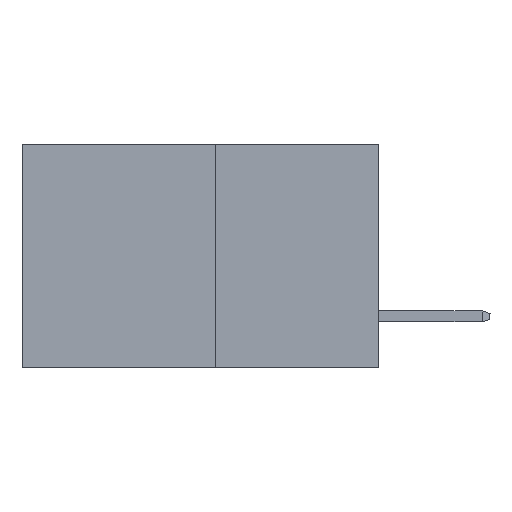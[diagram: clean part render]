
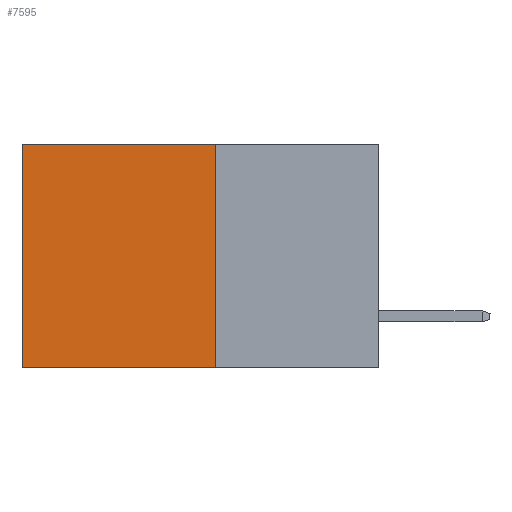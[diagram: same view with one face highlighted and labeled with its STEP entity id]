
A CAD part, left-side view. The second image highlights one B-rep face of the part: STEP entity #7595.
In plain terms, the highlighted planar face has unit normal (-1, 0, 0).
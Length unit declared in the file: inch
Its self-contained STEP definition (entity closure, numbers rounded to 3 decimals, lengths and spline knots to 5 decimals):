
#666 = CARTESIAN_POINT ( 'NONE',  ( 0.277, 0.59, -0.37 ) ) ;
#1176 = ORIENTED_EDGE ( 'NONE', *, *, #9642, .T. ) ;
#1651 = DIRECTION ( 'NONE',  ( 1., 0., 0. ) ) ;
#1742 = CARTESIAN_POINT ( 'NONE',  ( 0.277, 0.27, -0.37 ) ) ;
#2065 = LINE ( 'NONE', #10986, #4823 ) ;
#2217 = VECTOR ( 'NONE', #12589, 39.37008 ) ;
#2310 = EDGE_CURVE ( 'NONE', #8535, #12122, #2065, .T. ) ;
#2822 = CARTESIAN_POINT ( 'NONE',  ( 0.277, 0.59, 0. ) ) ;
#3288 = EDGE_CURVE ( 'NONE', #3587, #8535, #10731, .T. ) ;
#3301 = ORIENTED_EDGE ( 'NONE', *, *, #3288, .F. ) ;
#3587 = VERTEX_POINT ( 'NONE', #5481 ) ;
#4823 = VECTOR ( 'NONE', #12206, 39.37008 ) ;
#5037 = FACE_OUTER_BOUND ( 'NONE', #9085, .T. ) ;
#5169 = VECTOR ( 'NONE', #5943, 39.37008 ) ;
#5481 = CARTESIAN_POINT ( 'NONE',  ( 0.277, 0.27, 0. ) ) ;
#5796 = CARTESIAN_POINT ( 'NONE',  ( 0.277, 0.27, -0.37 ) ) ;
#5943 = DIRECTION ( 'NONE',  ( 0., 1., 0. ) ) ;
#6139 = CARTESIAN_POINT ( 'NONE',  ( 0.277, 0.27, -0.37 ) ) ;
#6312 = CARTESIAN_POINT ( 'NONE',  ( 0.277, 0.59, -0.37 ) ) ;
#6436 = ORIENTED_EDGE ( 'NONE', *, *, #2310, .F. ) ;
#7314 = ORIENTED_EDGE ( 'NONE', *, *, #11228, .T. ) ;
#7595 = ADVANCED_FACE ( 'NONE', ( #5037 ), #8092, .F. ) ;
#8092 = PLANE ( 'NONE',  #11767 ) ;
#8535 = VERTEX_POINT ( 'NONE', #1742 ) ;
#9043 = DIRECTION ( 'NONE',  ( 0., 0., -1. ) ) ;
#9085 = EDGE_LOOP ( 'NONE', ( #7314, #6436, #3301, #1176 ) ) ;
#9161 = VECTOR ( 'NONE', #11234, 39.37008 ) ;
#9642 = EDGE_CURVE ( 'NONE', #3587, #9860, #12804, .T. ) ;
#9860 = VERTEX_POINT ( 'NONE', #2822 ) ;
#10720 = CARTESIAN_POINT ( 'NONE',  ( 0.277, 0.27, 0. ) ) ;
#10731 = LINE ( 'NONE', #5796, #2217 ) ;
#10828 = LINE ( 'NONE', #666, #9161 ) ;
#10986 = CARTESIAN_POINT ( 'NONE',  ( 0.277, 0.27, -0.37 ) ) ;
#11228 = EDGE_CURVE ( 'NONE', #9860, #12122, #10828, .T. ) ;
#11234 = DIRECTION ( 'NONE',  ( 0., 0., -1. ) ) ;
#11767 = AXIS2_PLACEMENT_3D ( 'NONE', #6139, #1651, #9043 ) ;
#12122 = VERTEX_POINT ( 'NONE', #6312 ) ;
#12206 = DIRECTION ( 'NONE',  ( 0., 1., 0. ) ) ;
#12589 = DIRECTION ( 'NONE',  ( 0., 0., -1. ) ) ;
#12804 = LINE ( 'NONE', #10720, #5169 ) ;
